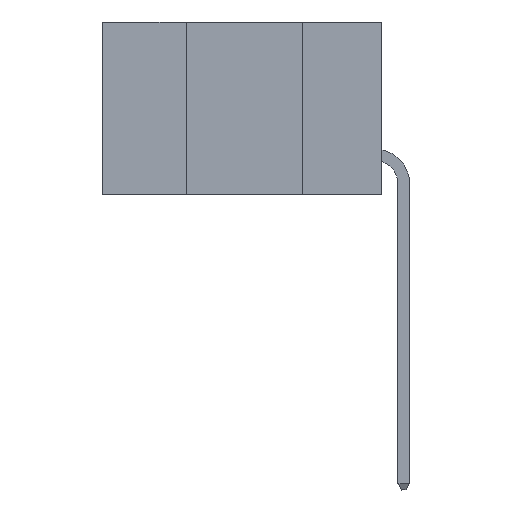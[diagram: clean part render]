
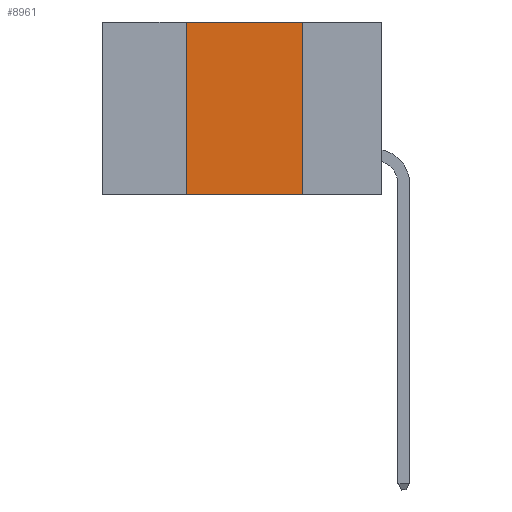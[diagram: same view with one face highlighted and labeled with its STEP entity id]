
A CAD part, left-side view. The second image highlights one B-rep face of the part: STEP entity #8961.
In plain terms, the highlighted planar face has unit normal (-1, 0, 0).
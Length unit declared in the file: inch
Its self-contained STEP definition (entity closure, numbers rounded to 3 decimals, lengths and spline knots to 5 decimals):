
#161 = EDGE_CURVE ( 'NONE', #24008, #12691, #26692, .T. ) ;
#833 = ORIENTED_EDGE ( 'NONE', *, *, #40950, .F. ) ;
#1001 = DIRECTION ( 'NONE',  ( 0., 0., 1. ) ) ;
#3939 = LINE ( 'NONE', #24467, #20170 ) ;
#4069 = VECTOR ( 'NONE', #4917, 39.37008 ) ;
#4917 = DIRECTION ( 'NONE',  ( 0., -1., 0. ) ) ;
#7051 = VECTOR ( 'NONE', #1001, 39.37008 ) ;
#8961 = ADVANCED_FACE ( 'NONE', ( #19664 ), #40597, .F. ) ;
#9091 = CARTESIAN_POINT ( 'NONE',  ( 0., 0.42, 0. ) ) ;
#9832 = CARTESIAN_POINT ( 'NONE',  ( 0., 0.17, -0.37 ) ) ;
#10861 = LINE ( 'NONE', #45967, #27071 ) ;
#12469 = CARTESIAN_POINT ( 'NONE',  ( 0., 0.42, 0. ) ) ;
#12691 = VERTEX_POINT ( 'NONE', #12469 ) ;
#13740 = EDGE_LOOP ( 'NONE', ( #38562, #833, #35297, #15393 ) ) ;
#15393 = ORIENTED_EDGE ( 'NONE', *, *, #34108, .T. ) ;
#19664 = FACE_OUTER_BOUND ( 'NONE', #13740, .T. ) ;
#20170 = VECTOR ( 'NONE', #35843, 39.37008 ) ;
#24008 = VERTEX_POINT ( 'NONE', #33132 ) ;
#24467 = CARTESIAN_POINT ( 'NONE',  ( 0., 0.6, -0.37 ) ) ;
#25865 = DIRECTION ( 'NONE',  ( 1., 0., 0. ) ) ;
#26692 = LINE ( 'NONE', #9091, #7051 ) ;
#27071 = VECTOR ( 'NONE', #34651, 39.37008 ) ;
#28786 = EDGE_CURVE ( 'NONE', #32531, #37980, #10861, .T. ) ;
#32531 = VERTEX_POINT ( 'NONE', #47967 ) ;
#33132 = CARTESIAN_POINT ( 'NONE',  ( 0., 0.42, -0.37 ) ) ;
#34108 = EDGE_CURVE ( 'NONE', #24008, #37980, #3939, .T. ) ;
#34178 = LINE ( 'NONE', #38595, #4069 ) ;
#34651 = DIRECTION ( 'NONE',  ( 0., 0., -1. ) ) ;
#35297 = ORIENTED_EDGE ( 'NONE', *, *, #161, .F. ) ;
#35843 = DIRECTION ( 'NONE',  ( 0., -1., 0. ) ) ;
#37980 = VERTEX_POINT ( 'NONE', #9832 ) ;
#38562 = ORIENTED_EDGE ( 'NONE', *, *, #28786, .F. ) ;
#38595 = CARTESIAN_POINT ( 'NONE',  ( 0., 0.6, 0. ) ) ;
#40597 = PLANE ( 'NONE',  #42800 ) ;
#40950 = EDGE_CURVE ( 'NONE', #12691, #32531, #34178, .T. ) ;
#41380 = DIRECTION ( 'NONE',  ( 0., 0., -1. ) ) ;
#42800 = AXIS2_PLACEMENT_3D ( 'NONE', #44297, #25865, #41380 ) ;
#44297 = CARTESIAN_POINT ( 'NONE',  ( 0., 0.6, 0. ) ) ;
#45967 = CARTESIAN_POINT ( 'NONE',  ( 0., 0.17, 0. ) ) ;
#47967 = CARTESIAN_POINT ( 'NONE',  ( 0., 0.17, 0. ) ) ;
